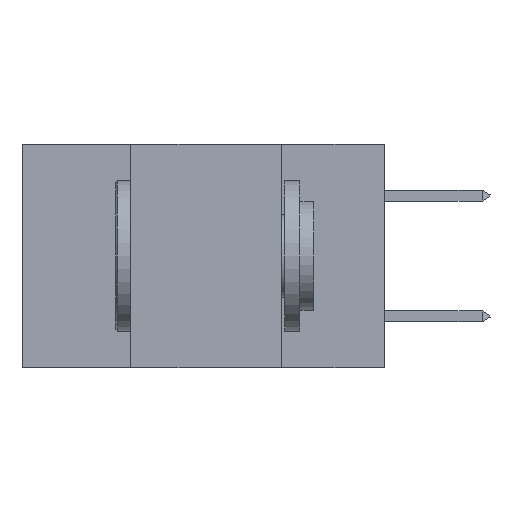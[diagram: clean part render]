
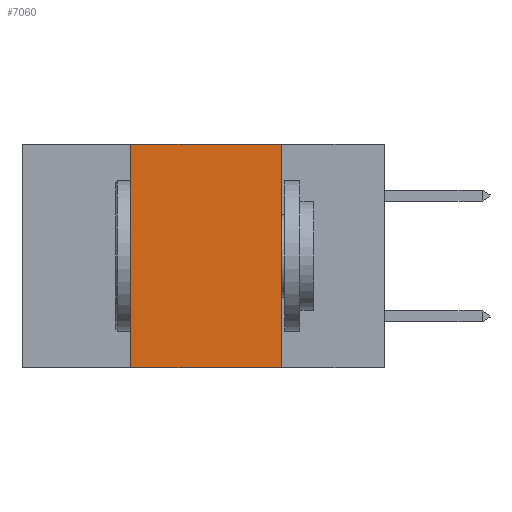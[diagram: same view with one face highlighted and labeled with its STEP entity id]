
A CAD part, left-side view. The second image highlights one B-rep face of the part: STEP entity #7060.
In plain terms, the highlighted planar face has unit normal (-1, 0, 0).
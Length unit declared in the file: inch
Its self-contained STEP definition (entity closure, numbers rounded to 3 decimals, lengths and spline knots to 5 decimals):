
#1348 = ORIENTED_EDGE ( 'NONE', *, *, #23476, .F. ) ;
#1439 = VERTEX_POINT ( 'NONE', #4370 ) ;
#1548 = CARTESIAN_POINT ( 'NONE',  ( 0., 0.17, -0.37 ) ) ;
#1664 = EDGE_CURVE ( 'NONE', #1439, #36546, #30994, .T. ) ;
#4370 = CARTESIAN_POINT ( 'NONE',  ( 0., 0.17, 0. ) ) ;
#4930 = CARTESIAN_POINT ( 'NONE',  ( 0., 0.6, 0. ) ) ;
#6854 = DIRECTION ( 'NONE',  ( 0., -1., 0. ) ) ;
#6996 = CARTESIAN_POINT ( 'NONE',  ( 0., 0.42, 0. ) ) ;
#7060 = ADVANCED_FACE ( 'NONE', ( #9926 ), #10533, .F. ) ;
#7489 = ORIENTED_EDGE ( 'NONE', *, *, #19870, .F. ) ;
#8405 = VECTOR ( 'NONE', #29852, 39.37008 ) ;
#9133 = LINE ( 'NONE', #4930, #30724 ) ;
#9926 = FACE_OUTER_BOUND ( 'NONE', #13630, .T. ) ;
#10533 = PLANE ( 'NONE',  #26158 ) ;
#10894 = LINE ( 'NONE', #29847, #32460 ) ;
#12645 = ORIENTED_EDGE ( 'NONE', *, *, #1664, .F. ) ;
#13630 = EDGE_LOOP ( 'NONE', ( #12645, #1348, #7489, #32611 ) ) ;
#15595 = EDGE_CURVE ( 'NONE', #19321, #36546, #10894, .T. ) ;
#15847 = DIRECTION ( 'NONE',  ( 0., -1., 0. ) ) ;
#19321 = VERTEX_POINT ( 'NONE', #32229 ) ;
#19870 = EDGE_CURVE ( 'NONE', #19321, #23843, #26391, .T. ) ;
#21359 = CARTESIAN_POINT ( 'NONE',  ( 0., 0.6, 0. ) ) ;
#21525 = CARTESIAN_POINT ( 'NONE',  ( 0., 0.17, 0. ) ) ;
#23476 = EDGE_CURVE ( 'NONE', #23843, #1439, #9133, .T. ) ;
#23843 = VERTEX_POINT ( 'NONE', #32780 ) ;
#26158 = AXIS2_PLACEMENT_3D ( 'NONE', #21359, #27740, #27877 ) ;
#26391 = LINE ( 'NONE', #6996, #8405 ) ;
#27740 = DIRECTION ( 'NONE',  ( 1., 0., 0. ) ) ;
#27877 = DIRECTION ( 'NONE',  ( 0., 0., -1. ) ) ;
#29847 = CARTESIAN_POINT ( 'NONE',  ( 0., 0.6, -0.37 ) ) ;
#29852 = DIRECTION ( 'NONE',  ( 0., 0., 1. ) ) ;
#30111 = VECTOR ( 'NONE', #32409, 39.37008 ) ;
#30724 = VECTOR ( 'NONE', #15847, 39.37008 ) ;
#30994 = LINE ( 'NONE', #21525, #30111 ) ;
#32229 = CARTESIAN_POINT ( 'NONE',  ( 0., 0.42, -0.37 ) ) ;
#32409 = DIRECTION ( 'NONE',  ( 0., 0., -1. ) ) ;
#32460 = VECTOR ( 'NONE', #6854, 39.37008 ) ;
#32611 = ORIENTED_EDGE ( 'NONE', *, *, #15595, .T. ) ;
#32780 = CARTESIAN_POINT ( 'NONE',  ( 0., 0.42, 0. ) ) ;
#36546 = VERTEX_POINT ( 'NONE', #1548 ) ;
